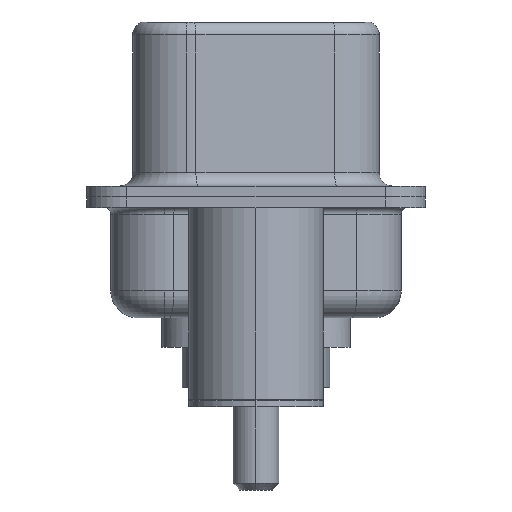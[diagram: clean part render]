
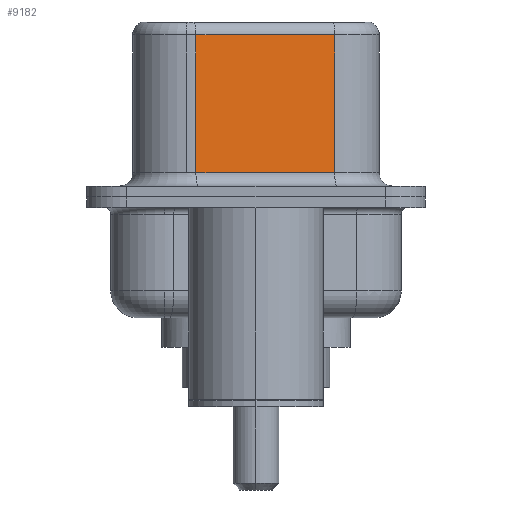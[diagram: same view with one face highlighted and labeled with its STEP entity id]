
A CAD part, left-side view. The second image highlights one B-rep face of the part: STEP entity #9182.
In plain terms, the highlighted planar face has unit normal (-0.985, -0.174, 0).
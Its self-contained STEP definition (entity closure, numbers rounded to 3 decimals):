
#767 = PLANE ( 'NONE',  #18489 ) ;
#785 = DIRECTION ( 'NONE',  ( -0.174, 0.985, 0. ) ) ;
#1503 = ORIENTED_EDGE ( 'NONE', *, *, #5394, .F. ) ;
#1553 = FACE_OUTER_BOUND ( 'NONE', #15431, .T. ) ;
#2091 = CARTESIAN_POINT ( 'NONE',  ( 3.67, 2.233, 0.9 ) ) ;
#2329 = VECTOR ( 'NONE', #10490, 1000. ) ;
#2675 = ORIENTED_EDGE ( 'NONE', *, *, #15344, .T. ) ;
#4452 = EDGE_CURVE ( 'NONE', #6224, #16044, #9843, .T. ) ;
#4760 = CARTESIAN_POINT ( 'NONE',  ( 4.58, -2.927, 0.9 ) ) ;
#5394 = EDGE_CURVE ( 'NONE', #11120, #16044, #18066, .T. ) ;
#5419 = DIRECTION ( 'NONE',  ( 0., 0., -1. ) ) ;
#6224 = VERTEX_POINT ( 'NONE', #2091 ) ;
#6877 = VECTOR ( 'NONE', #5419, 1000. ) ;
#8158 = LINE ( 'NONE', #10411, #9697 ) ;
#9182 = ADVANCED_FACE ( 'NONE', ( #1553 ), #767, .F. ) ;
#9697 = VECTOR ( 'NONE', #9931, 1000. ) ;
#9843 = LINE ( 'NONE', #14520, #2329 ) ;
#9931 = DIRECTION ( 'NONE',  ( -0.174, 0.985, 0. ) ) ;
#10411 = CARTESIAN_POINT ( 'NONE',  ( 4.58, -2.927, 6.02 ) ) ;
#10490 = DIRECTION ( 'NONE',  ( 0.174, -0.985, 0. ) ) ;
#10735 = EDGE_CURVE ( 'NONE', #11120, #15308, #8158, .T. ) ;
#11058 = ORIENTED_EDGE ( 'NONE', *, *, #10735, .T. ) ;
#11120 = VERTEX_POINT ( 'NONE', #16533 ) ;
#13073 = DIRECTION ( 'NONE',  ( 0.985, 0.174, 0. ) ) ;
#13308 = DIRECTION ( 'NONE',  ( 0., 0., -1. ) ) ;
#13796 = VECTOR ( 'NONE', #13308, 1000. ) ;
#13884 = CARTESIAN_POINT ( 'NONE',  ( 3.67, 2.233, 6.52 ) ) ;
#14373 = LINE ( 'NONE', #13884, #6877 ) ;
#14520 = CARTESIAN_POINT ( 'NONE',  ( 4.58, -2.927, 0.9 ) ) ;
#14580 = ORIENTED_EDGE ( 'NONE', *, *, #4452, .T. ) ;
#15200 = CARTESIAN_POINT ( 'NONE',  ( 4.58, -2.927, 6.52 ) ) ;
#15308 = VERTEX_POINT ( 'NONE', #16645 ) ;
#15344 = EDGE_CURVE ( 'NONE', #15308, #6224, #14373, .T. ) ;
#15431 = EDGE_LOOP ( 'NONE', ( #1503, #11058, #2675, #14580 ) ) ;
#15698 = CARTESIAN_POINT ( 'NONE',  ( 4.58, -2.927, 6.52 ) ) ;
#16044 = VERTEX_POINT ( 'NONE', #4760 ) ;
#16533 = CARTESIAN_POINT ( 'NONE',  ( 4.58, -2.927, 6.02 ) ) ;
#16645 = CARTESIAN_POINT ( 'NONE',  ( 3.67, 2.233, 6.02 ) ) ;
#18066 = LINE ( 'NONE', #15698, #13796 ) ;
#18489 = AXIS2_PLACEMENT_3D ( 'NONE', #15200, #13073, #785 ) ;
